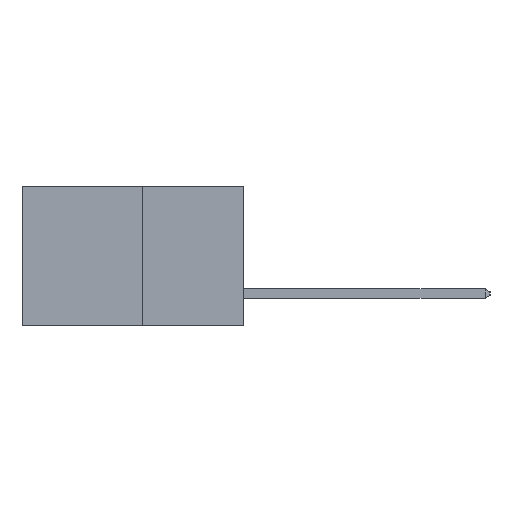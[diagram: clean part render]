
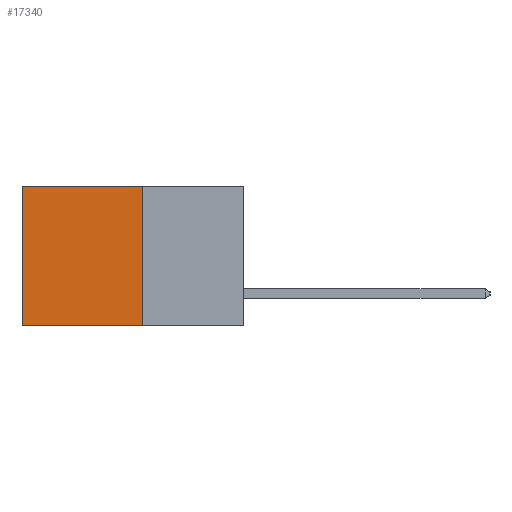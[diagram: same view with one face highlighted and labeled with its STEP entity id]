
A CAD part, left-side view. The second image highlights one B-rep face of the part: STEP entity #17340.
In plain terms, the highlighted planar face has unit normal (-1, 0, 0).
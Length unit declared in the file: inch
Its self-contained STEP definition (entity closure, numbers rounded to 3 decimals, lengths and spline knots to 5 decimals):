
#1142 = ORIENTED_EDGE ( 'NONE', *, *, #11968, .F. ) ;
#3365 = CARTESIAN_POINT ( 'NONE',  ( 0.277, 0.59, -0.37 ) ) ;
#4182 = VECTOR ( 'NONE', #21668, 39.37008 ) ;
#4212 = VERTEX_POINT ( 'NONE', #13688 ) ;
#4855 = VECTOR ( 'NONE', #5603, 39.37008 ) ;
#5076 = ORIENTED_EDGE ( 'NONE', *, *, #23643, .T. ) ;
#5603 = DIRECTION ( 'NONE',  ( 0., 0., -1. ) ) ;
#6463 = CARTESIAN_POINT ( 'NONE',  ( 0.277, 0.59, 0. ) ) ;
#7414 = CARTESIAN_POINT ( 'NONE',  ( 0.277, 0.59, -0.37 ) ) ;
#9210 = CARTESIAN_POINT ( 'NONE',  ( 0.277, 0.27, -0.37 ) ) ;
#9764 = ORIENTED_EDGE ( 'NONE', *, *, #27756, .F. ) ;
#11338 = DIRECTION ( 'NONE',  ( 1., 0., 0. ) ) ;
#11796 = VERTEX_POINT ( 'NONE', #6463 ) ;
#11968 = EDGE_CURVE ( 'NONE', #4212, #24410, #12910, .T. ) ;
#12372 = CARTESIAN_POINT ( 'NONE',  ( 0.277, 0.27, -0.37 ) ) ;
#12910 = LINE ( 'NONE', #9210, #19383 ) ;
#12943 = CARTESIAN_POINT ( 'NONE',  ( 0.277, 0.27, -0.37 ) ) ;
#12985 = CARTESIAN_POINT ( 'NONE',  ( 0.277, 0.27, 0. ) ) ;
#13474 = EDGE_LOOP ( 'NONE', ( #5076, #9764, #1142, #16329 ) ) ;
#13688 = CARTESIAN_POINT ( 'NONE',  ( 0.277, 0.27, 0. ) ) ;
#16104 = EDGE_CURVE ( 'NONE', #4212, #11796, #20699, .T. ) ;
#16214 = FACE_OUTER_BOUND ( 'NONE', #13474, .T. ) ;
#16329 = ORIENTED_EDGE ( 'NONE', *, *, #16104, .T. ) ;
#16417 = LINE ( 'NONE', #3365, #4855 ) ;
#17340 = ADVANCED_FACE ( 'NONE', ( #16214 ), #19401, .F. ) ;
#19173 = AXIS2_PLACEMENT_3D ( 'NONE', #24313, #11338, #26492 ) ;
#19383 = VECTOR ( 'NONE', #24333, 39.37008 ) ;
#19401 = PLANE ( 'NONE',  #19173 ) ;
#20651 = VERTEX_POINT ( 'NONE', #7414 ) ;
#20699 = LINE ( 'NONE', #12985, #25778 ) ;
#21668 = DIRECTION ( 'NONE',  ( 0., 1., 0. ) ) ;
#22175 = LINE ( 'NONE', #12943, #4182 ) ;
#23643 = EDGE_CURVE ( 'NONE', #11796, #20651, #16417, .T. ) ;
#23790 = DIRECTION ( 'NONE',  ( 0., 1., 0. ) ) ;
#24313 = CARTESIAN_POINT ( 'NONE',  ( 0.277, 0.27, -0.37 ) ) ;
#24333 = DIRECTION ( 'NONE',  ( 0., 0., -1. ) ) ;
#24410 = VERTEX_POINT ( 'NONE', #12372 ) ;
#25778 = VECTOR ( 'NONE', #23790, 39.37008 ) ;
#26492 = DIRECTION ( 'NONE',  ( 0., 0., -1. ) ) ;
#27756 = EDGE_CURVE ( 'NONE', #24410, #20651, #22175, .T. ) ;
